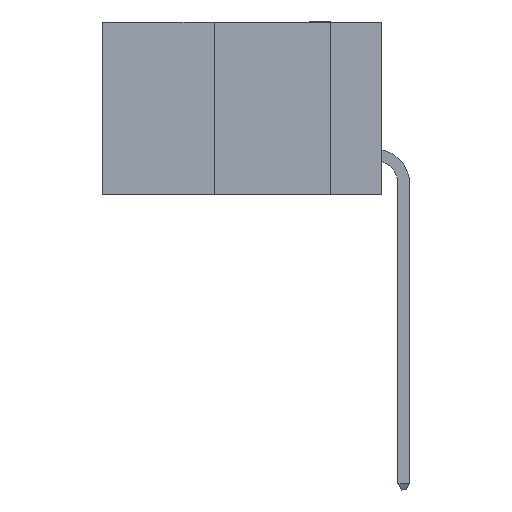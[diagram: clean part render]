
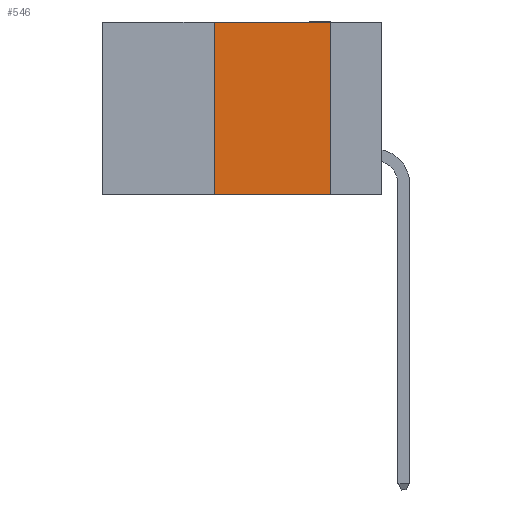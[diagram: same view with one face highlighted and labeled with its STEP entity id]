
A CAD part, left-side view. The second image highlights one B-rep face of the part: STEP entity #546.
In plain terms, the highlighted planar face has unit normal (-1, 0, 0).
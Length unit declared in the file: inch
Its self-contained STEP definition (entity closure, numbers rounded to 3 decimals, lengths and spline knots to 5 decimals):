
#356 = CARTESIAN_POINT ( 'NONE',  ( 0., 0.11, 0. ) ) ;
#546 = ADVANCED_FACE ( 'NONE', ( #14089 ), #1775, .F. ) ;
#705 = CARTESIAN_POINT ( 'NONE',  ( 0., 0.6, -0.37 ) ) ;
#721 = EDGE_LOOP ( 'NONE', ( #11783, #2277, #12529, #12367 ) ) ;
#1557 = VERTEX_POINT ( 'NONE', #356 ) ;
#1608 = CARTESIAN_POINT ( 'NONE',  ( 0., 0.6, 0. ) ) ;
#1775 = PLANE ( 'NONE',  #3037 ) ;
#2277 = ORIENTED_EDGE ( 'NONE', *, *, #11004, .F. ) ;
#2534 = CARTESIAN_POINT ( 'NONE',  ( 0., 0.36, 0. ) ) ;
#2729 = DIRECTION ( 'NONE',  ( 0., -1., 0. ) ) ;
#2809 = VERTEX_POINT ( 'NONE', #5252 ) ;
#3037 = AXIS2_PLACEMENT_3D ( 'NONE', #1608, #14358, #14339 ) ;
#4998 = EDGE_CURVE ( 'NONE', #1557, #5270, #13167, .T. ) ;
#5252 = CARTESIAN_POINT ( 'NONE',  ( 0., 0.36, -0.37 ) ) ;
#5270 = VERTEX_POINT ( 'NONE', #9025 ) ;
#5728 = DIRECTION ( 'NONE',  ( 0., 0., 1. ) ) ;
#7288 = VERTEX_POINT ( 'NONE', #2534 ) ;
#7555 = EDGE_CURVE ( 'NONE', #2809, #7288, #15534, .T. ) ;
#8282 = VECTOR ( 'NONE', #2729, 39.37008 ) ;
#8412 = EDGE_CURVE ( 'NONE', #2809, #5270, #14828, .T. ) ;
#8744 = VECTOR ( 'NONE', #9795, 39.37008 ) ;
#9025 = CARTESIAN_POINT ( 'NONE',  ( 0., 0.11, -0.37 ) ) ;
#9795 = DIRECTION ( 'NONE',  ( 0., -1., 0. ) ) ;
#9953 = VECTOR ( 'NONE', #11127, 39.37008 ) ;
#10202 = CARTESIAN_POINT ( 'NONE',  ( 0., 0.11, 0. ) ) ;
#10379 = CARTESIAN_POINT ( 'NONE',  ( 0., 0.6, 0. ) ) ;
#11004 = EDGE_CURVE ( 'NONE', #7288, #1557, #14399, .T. ) ;
#11127 = DIRECTION ( 'NONE',  ( 0., 0., -1. ) ) ;
#11783 = ORIENTED_EDGE ( 'NONE', *, *, #4998, .F. ) ;
#12367 = ORIENTED_EDGE ( 'NONE', *, *, #8412, .T. ) ;
#12529 = ORIENTED_EDGE ( 'NONE', *, *, #7555, .F. ) ;
#12761 = VECTOR ( 'NONE', #5728, 39.37008 ) ;
#13154 = CARTESIAN_POINT ( 'NONE',  ( 0., 0.36, 0. ) ) ;
#13167 = LINE ( 'NONE', #10202, #9953 ) ;
#14089 = FACE_OUTER_BOUND ( 'NONE', #721, .T. ) ;
#14339 = DIRECTION ( 'NONE',  ( 0., 0., -1. ) ) ;
#14358 = DIRECTION ( 'NONE',  ( 1., 0., 0. ) ) ;
#14399 = LINE ( 'NONE', #10379, #8282 ) ;
#14828 = LINE ( 'NONE', #705, #8744 ) ;
#15534 = LINE ( 'NONE', #13154, #12761 ) ;
